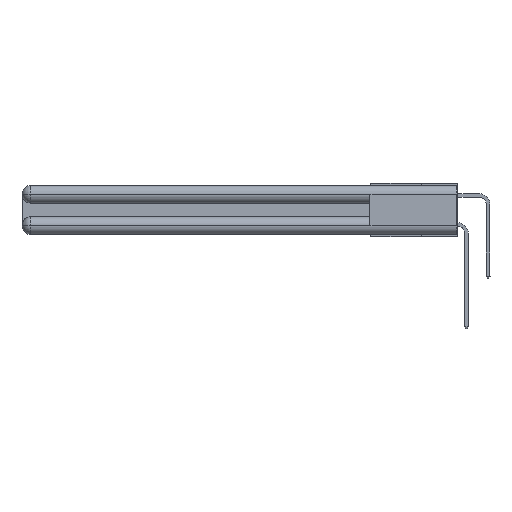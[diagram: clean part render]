
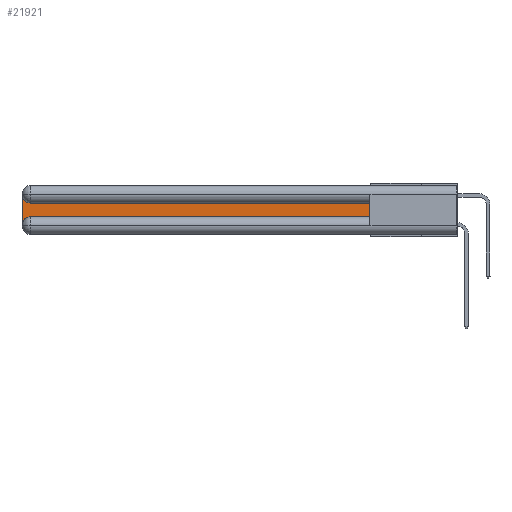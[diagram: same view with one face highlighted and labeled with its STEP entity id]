
A CAD part, left-side view. The second image highlights one B-rep face of the part: STEP entity #21921.
In plain terms, the highlighted planar face has unit normal (-1, 0, 0).
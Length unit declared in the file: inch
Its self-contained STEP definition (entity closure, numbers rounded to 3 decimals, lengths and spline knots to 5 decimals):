
#15 = VECTOR ( 'NONE', #31842, 39.37008 ) ;
#1955 = AXIS2_PLACEMENT_3D ( 'NONE', #20074, #10620, #5367 ) ;
#2087 = CARTESIAN_POINT ( 'NONE',  ( 0.075, 2.94, -0.2775 ) ) ;
#2813 = DIRECTION ( 'NONE',  ( 0., 0., -1. ) ) ;
#2900 = DIRECTION ( 'NONE',  ( 0., 0., -1. ) ) ;
#3024 = CIRCLE ( 'NONE', #4580, 0.06 ) ;
#3721 = ORIENTED_EDGE ( 'NONE', *, *, #23119, .T. ) ;
#4004 = CARTESIAN_POINT ( 'NONE',  ( 0.075, 0.6, -0.1225 ) ) ;
#4580 = AXIS2_PLACEMENT_3D ( 'NONE', #10107, #17809, #2813 ) ;
#4740 = CIRCLE ( 'NONE', #5196, 0.06 ) ;
#5196 = AXIS2_PLACEMENT_3D ( 'NONE', #2087, #12297, #9791 ) ;
#5367 = DIRECTION ( 'NONE',  ( 0., 0., -1. ) ) ;
#6214 = LINE ( 'NONE', #24387, #29682 ) ;
#6851 = CARTESIAN_POINT ( 'NONE',  ( 0.075, 0.6, -0.1225 ) ) ;
#7601 = VECTOR ( 'NONE', #2900, 39.37008 ) ;
#8579 = EDGE_CURVE ( 'NONE', #23343, #14374, #3024, .T. ) ;
#8652 = LINE ( 'NONE', #4004, #20573 ) ;
#9698 = CARTESIAN_POINT ( 'NONE',  ( 0.075, 0.6, -0.2175 ) ) ;
#9791 = DIRECTION ( 'NONE',  ( 0., 0., -1. ) ) ;
#10107 = CARTESIAN_POINT ( 'NONE',  ( 0.075, 2.94, -0.0625 ) ) ;
#10620 = DIRECTION ( 'NONE',  ( 1., 0., 0. ) ) ;
#10921 = VERTEX_POINT ( 'NONE', #9698 ) ;
#12297 = DIRECTION ( 'NONE',  ( 1., 0., 0. ) ) ;
#12370 = ORIENTED_EDGE ( 'NONE', *, *, #19943, .T. ) ;
#13636 = DIRECTION ( 'NONE',  ( 0., 1., 0. ) ) ;
#14173 = CARTESIAN_POINT ( 'NONE',  ( 0.075, 3., -0.0625 ) ) ;
#14374 = VERTEX_POINT ( 'NONE', #14173 ) ;
#17107 = ORIENTED_EDGE ( 'NONE', *, *, #8579, .T. ) ;
#17610 = ORIENTED_EDGE ( 'NONE', *, *, #27304, .T. ) ;
#17809 = DIRECTION ( 'NONE',  ( 1., 0., 0. ) ) ;
#19412 = EDGE_CURVE ( 'NONE', #20768, #10921, #6214, .T. ) ;
#19943 = EDGE_CURVE ( 'NONE', #10921, #30317, #29609, .T. ) ;
#20074 = CARTESIAN_POINT ( 'NONE',  ( 0.075, 3., -0.1225 ) ) ;
#20076 = EDGE_LOOP ( 'NONE', ( #3721, #17107, #17610, #24061, #29477, #12370 ) ) ;
#20399 = PLANE ( 'NONE',  #1955 ) ;
#20573 = VECTOR ( 'NONE', #13636, 39.37008 ) ;
#20768 = VERTEX_POINT ( 'NONE', #23054 ) ;
#21921 = ADVANCED_FACE ( 'NONE', ( #22189 ), #20399, .F. ) ;
#22189 = FACE_OUTER_BOUND ( 'NONE', #20076, .T. ) ;
#22222 = CARTESIAN_POINT ( 'NONE',  ( 0.075, 3., -0.2775 ) ) ;
#22681 = CARTESIAN_POINT ( 'NONE',  ( 0.075, 3., -0.2175 ) ) ;
#23054 = CARTESIAN_POINT ( 'NONE',  ( 0.075, 2.94, -0.2175 ) ) ;
#23119 = EDGE_CURVE ( 'NONE', #30317, #23343, #8652, .T. ) ;
#23343 = VERTEX_POINT ( 'NONE', #24760 ) ;
#24061 = ORIENTED_EDGE ( 'NONE', *, *, #31782, .T. ) ;
#24387 = CARTESIAN_POINT ( 'NONE',  ( 0.075, 0.6, -0.2175 ) ) ;
#24760 = CARTESIAN_POINT ( 'NONE',  ( 0.075, 2.94, -0.1225 ) ) ;
#26041 = LINE ( 'NONE', #22681, #7601 ) ;
#26766 = DIRECTION ( 'NONE',  ( 0., -1., 0. ) ) ;
#27304 = EDGE_CURVE ( 'NONE', #14374, #30342, #26041, .T. ) ;
#29477 = ORIENTED_EDGE ( 'NONE', *, *, #19412, .T. ) ;
#29609 = LINE ( 'NONE', #31725, #15 ) ;
#29682 = VECTOR ( 'NONE', #26766, 39.37008 ) ;
#30317 = VERTEX_POINT ( 'NONE', #6851 ) ;
#30342 = VERTEX_POINT ( 'NONE', #22222 ) ;
#31725 = CARTESIAN_POINT ( 'NONE',  ( 0.075, 0.6, -0.2175 ) ) ;
#31782 = EDGE_CURVE ( 'NONE', #30342, #20768, #4740, .T. ) ;
#31842 = DIRECTION ( 'NONE',  ( 0., 0., 1. ) ) ;
